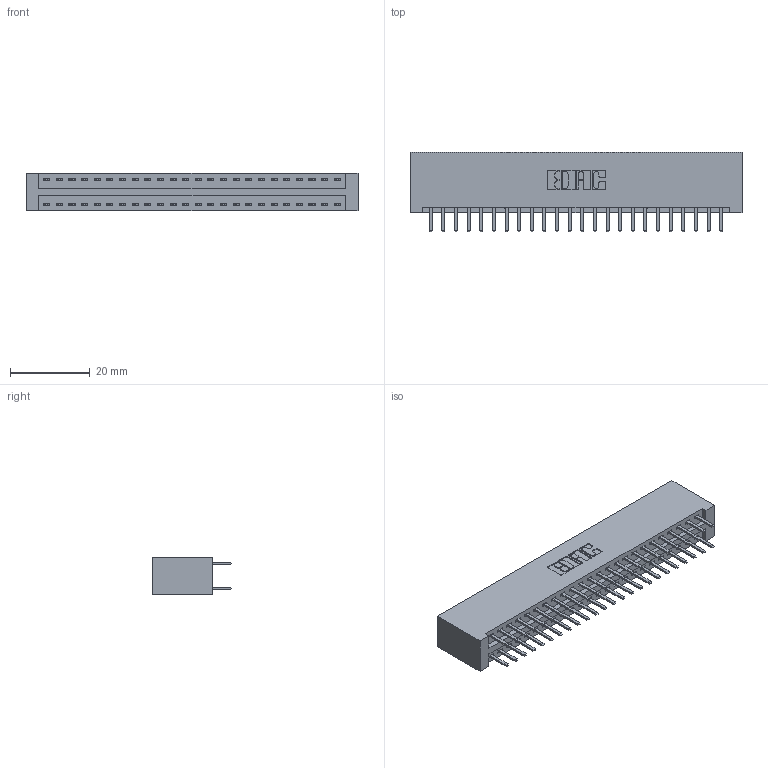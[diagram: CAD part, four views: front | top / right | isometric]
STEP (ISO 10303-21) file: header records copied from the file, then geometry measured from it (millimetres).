
FILE_DESCRIPTION (( 'STEP AP203' ), '1' );
FILE_NAME ('346-048-520-201.STEP', '2022-05-20T20:57:45', ( '' ), ( '' ), 'SwSTEP 2.0', 'SolidWorks 2020', '' );
FILE_SCHEMA (( 'CONFIG_CONTROL_DESIGN' ));
Length unit declared in the file: inch
Products named in the file (3): 346 Part_No Mounting Lugs; 346-048-520-201; 345-292-001_345-293-120
Assembly tree (49 placements, depth 2):
  346-048-520-201
    346 Part_No Mounting Lugs
    345-292-001_345-293-120  x48
Bounding box: 83.44 x 20.02 x 9.4 mm (x, y, z)
Volume: 8548.7 mm3; surface area: 11581.6 mm2
Topology: 49 solids, 49 shells, 2802 faces, 8129 edges, 5290 vertices
Faces by surface type: plane 1848, cylinder 954
Entity records: 17923 total; most frequent: CARTESIAN_POINT 2988, ORIENTED_EDGE 2910, DIRECTION 2667, EDGE_CURVE 1455, VECTOR 1231, LINE 1231, VERTEX_POINT 966, AXIS2_PLACEMENT_3D 718
